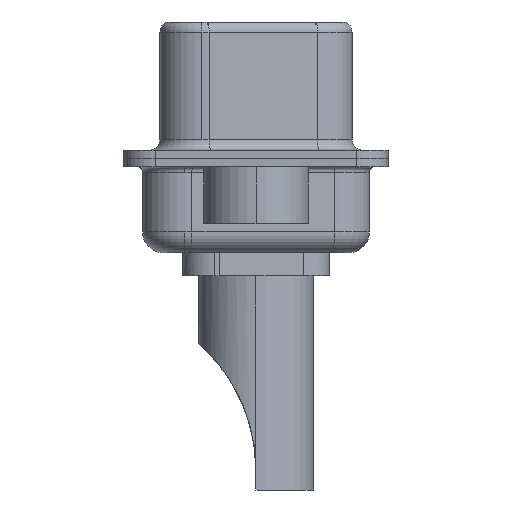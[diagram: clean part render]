
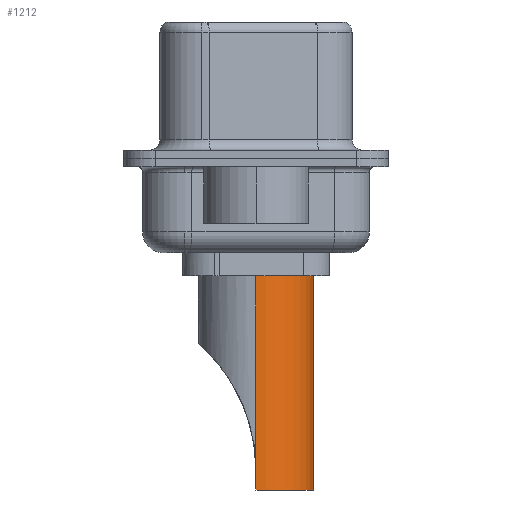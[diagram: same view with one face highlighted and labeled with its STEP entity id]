
A CAD part, left-side view. The second image highlights one B-rep face of the part: STEP entity #1212.
In plain terms, the highlighted cylindrical face has radius 2.75 mm (diameter 5.5 mm), a partial arc.
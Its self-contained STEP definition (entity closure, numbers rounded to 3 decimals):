
#91 = DIRECTION ( 'NONE',  ( 0., 0., -1. ) ) ;
#344 = CARTESIAN_POINT ( 'NONE',  ( -2.75, 0., 4.234 ) ) ;
#851 = DIRECTION ( 'NONE',  ( 0., 0., 1. ) ) ;
#1212 = ADVANCED_FACE ( 'NONE', ( #9626 ), #9058, .T. ) ;
#1219 = EDGE_CURVE ( 'NONE', #5585, #17014, #18744, .T. ) ;
#3291 = VECTOR ( 'NONE', #11194, 1000. ) ;
#5126 = AXIS2_PLACEMENT_3D ( 'NONE', #5395, #18071, #7190 ) ;
#5314 = CARTESIAN_POINT ( 'NONE',  ( 2.75, 0., -8.7 ) ) ;
#5395 = CARTESIAN_POINT ( 'NONE',  ( 0., 0., -8.7 ) ) ;
#5585 = VERTEX_POINT ( 'NONE', #10954 ) ;
#6448 = CARTESIAN_POINT ( 'NONE',  ( 0., 0., 4.234 ) ) ;
#7190 = DIRECTION ( 'NONE',  ( 1., 0., 0. ) ) ;
#8416 = VERTEX_POINT ( 'NONE', #9342 ) ;
#8475 = CARTESIAN_POINT ( 'NONE',  ( 0., 0., 1.5 ) ) ;
#8625 = EDGE_CURVE ( 'NONE', #12882, #17014, #18987, .T. ) ;
#8941 = EDGE_CURVE ( 'NONE', #12123, #8416, #13275, .T. ) ;
#9058 = CYLINDRICAL_SURFACE ( 'NONE', #10956, 2.75 ) ;
#9342 = CARTESIAN_POINT ( 'NONE',  ( 2.75, 0., -8.7 ) ) ;
#9626 = FACE_OUTER_BOUND ( 'NONE', #14181, .T. ) ;
#9704 = CARTESIAN_POINT ( 'NONE',  ( -2.75, 0., -8.7 ) ) ;
#9713 = ORIENTED_EDGE ( 'NONE', *, *, #10748, .F. ) ;
#9735 = AXIS2_PLACEMENT_3D ( 'NONE', #8475, #15327, #10107 ) ;
#9881 = CARTESIAN_POINT ( 'NONE',  ( 2.75, 0., 4.234 ) ) ;
#10107 = DIRECTION ( 'NONE',  ( 1., 0., 0. ) ) ;
#10748 = EDGE_CURVE ( 'NONE', #21850, #5585, #17765, .T. ) ;
#10950 = CARTESIAN_POINT ( 'NONE',  ( -2.75, 0., -8.7 ) ) ;
#10954 = CARTESIAN_POINT ( 'NONE',  ( -2.75, 0., 1.5 ) ) ;
#10956 = AXIS2_PLACEMENT_3D ( 'NONE', #6448, #12683, #21492 ) ;
#10976 = CARTESIAN_POINT ( 'NONE',  ( 2.75, 0., 1.5 ) ) ;
#11194 = DIRECTION ( 'NONE',  ( 0., 0., 1. ) ) ;
#12123 = VERTEX_POINT ( 'NONE', #9704 ) ;
#12683 = DIRECTION ( 'NONE',  ( 0., 0., 1. ) ) ;
#12687 = LINE ( 'NONE', #10950, #22921 ) ;
#12882 = VERTEX_POINT ( 'NONE', #13806 ) ;
#13172 = ORIENTED_EDGE ( 'NONE', *, *, #21609, .T. ) ;
#13275 = CIRCLE ( 'NONE', #5126, 2.75 ) ;
#13806 = CARTESIAN_POINT ( 'NONE',  ( 2.75, 0., -7.764 ) ) ;
#14181 = EDGE_LOOP ( 'NONE', ( #9713, #13172, #22186, #15910, #19197, #14456 ) ) ;
#14456 = ORIENTED_EDGE ( 'NONE', *, *, #1219, .F. ) ;
#15094 = CARTESIAN_POINT ( 'NONE',  ( -2.75, 0., -7.764 ) ) ;
#15327 = DIRECTION ( 'NONE',  ( 0., 0., 1. ) ) ;
#15746 = EDGE_CURVE ( 'NONE', #12882, #8416, #17189, .T. ) ;
#15910 = ORIENTED_EDGE ( 'NONE', *, *, #15746, .F. ) ;
#17014 = VERTEX_POINT ( 'NONE', #10976 ) ;
#17189 = LINE ( 'NONE', #5314, #21471 ) ;
#17765 = LINE ( 'NONE', #344, #3291 ) ;
#18071 = DIRECTION ( 'NONE',  ( 0., 0., 1. ) ) ;
#18744 = CIRCLE ( 'NONE', #9735, 2.75 ) ;
#18987 = LINE ( 'NONE', #9881, #23233 ) ;
#19197 = ORIENTED_EDGE ( 'NONE', *, *, #8625, .T. ) ;
#19744 = DIRECTION ( 'NONE',  ( 0., 0., -1. ) ) ;
#21471 = VECTOR ( 'NONE', #19744, 1000. ) ;
#21492 = DIRECTION ( 'NONE',  ( 1., 0., 0. ) ) ;
#21609 = EDGE_CURVE ( 'NONE', #21850, #12123, #12687, .T. ) ;
#21850 = VERTEX_POINT ( 'NONE', #15094 ) ;
#22186 = ORIENTED_EDGE ( 'NONE', *, *, #8941, .T. ) ;
#22921 = VECTOR ( 'NONE', #91, 1000. ) ;
#23233 = VECTOR ( 'NONE', #851, 1000. ) ;
